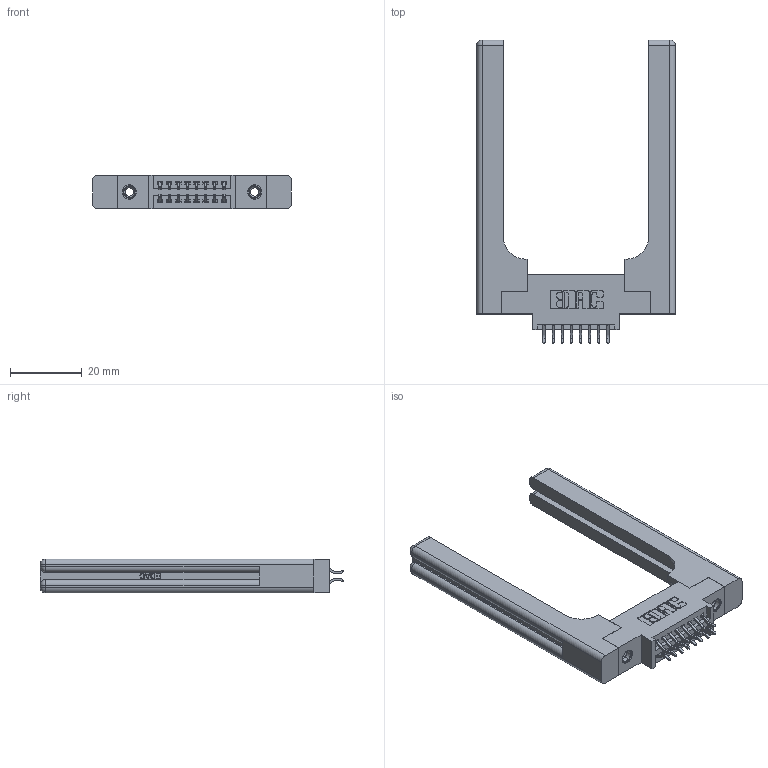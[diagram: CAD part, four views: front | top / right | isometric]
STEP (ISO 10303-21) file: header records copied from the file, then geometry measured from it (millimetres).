
FILE_DESCRIPTION (( 'STEP AP203' ), '1' );
FILE_NAME ('345-016-556-858.STEP', '2019-10-27T04:53:22', ( '' ), ( '' ), 'SwSTEP 2.0', 'SolidWorks 2016', '' );
FILE_SCHEMA (( 'CONFIG_CONTROL_DESIGN' ));
Length unit declared in the file: inch
Products named in the file (5): 345 Part_0.170 Offset - 0.156 Dia-TH; 345-292-001_556 Tail; 345-250-001_345-250-001-102; 345-220-058_345-220-058; 345-016-556-858
Assembly tree (21 placements, depth 2):
  345-016-556-858
    345 Part_0.170 Offset - 0.156 Dia-TH
    345-292-001_556 Tail  x16
    345-250-001_345-250-001-102  x2
    345-220-058_345-220-058  x2
Bounding box: 55.35 x 84.51 x 9.4 mm (x, y, z)
Volume: 13421.9 mm3; surface area: 11842 mm2
Topology: 21 solids, 21 shells, 1282 faces, 3691 edges, 2418 vertices
Faces by surface type: plane 824, cylinder 398, bspline 36, cone 12, sphere 8, torus 4
Entity records: 16388 total; most frequent: CARTESIAN_POINT 3789, ORIENTED_EDGE 2508, DIRECTION 2302, EDGE_CURVE 1254, VECTOR 990, LINE 990, VERTEX_POINT 826, AXIS2_PLACEMENT_3D 656
